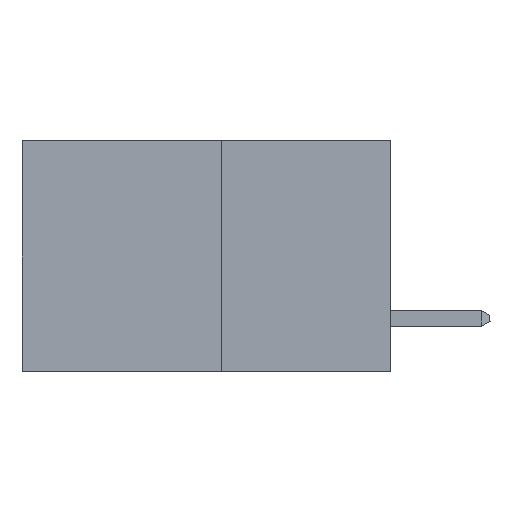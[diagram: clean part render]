
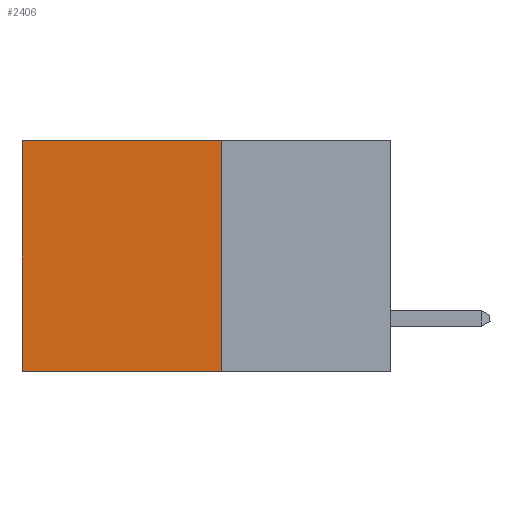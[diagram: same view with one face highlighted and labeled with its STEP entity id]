
A CAD part, left-side view. The second image highlights one B-rep face of the part: STEP entity #2406.
In plain terms, the highlighted planar face has unit normal (-1, 0, 0).
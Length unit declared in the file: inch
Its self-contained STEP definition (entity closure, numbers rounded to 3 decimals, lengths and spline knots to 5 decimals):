
#438 = VECTOR ( 'NONE', #16732, 39.37008 ) ;
#534 = VERTEX_POINT ( 'NONE', #14282 ) ;
#1206 = AXIS2_PLACEMENT_3D ( 'NONE', #14057, #15359, #7494 ) ;
#1408 = VECTOR ( 'NONE', #11348, 39.37008 ) ;
#2335 = CARTESIAN_POINT ( 'NONE',  ( 0.277, 0.27, -0.37 ) ) ;
#2406 = ADVANCED_FACE ( 'NONE', ( #8307 ), #11424, .F. ) ;
#2474 = ORIENTED_EDGE ( 'NONE', *, *, #8047, .T. ) ;
#2562 = DIRECTION ( 'NONE',  ( 0., 0., -1. ) ) ;
#2652 = VECTOR ( 'NONE', #2562, 39.37008 ) ;
#3081 = LINE ( 'NONE', #4979, #9716 ) ;
#3477 = VERTEX_POINT ( 'NONE', #4419 ) ;
#3604 = CARTESIAN_POINT ( 'NONE',  ( 0.277, 0.27, -0.37 ) ) ;
#3862 = CARTESIAN_POINT ( 'NONE',  ( 0.277, 0.59, -0.37 ) ) ;
#4419 = CARTESIAN_POINT ( 'NONE',  ( 0.277, 0.59, 0. ) ) ;
#4979 = CARTESIAN_POINT ( 'NONE',  ( 0.277, 0.59, -0.37 ) ) ;
#6320 = DIRECTION ( 'NONE',  ( 0., 0., -1. ) ) ;
#7274 = EDGE_CURVE ( 'NONE', #534, #3477, #8910, .T. ) ;
#7480 = VERTEX_POINT ( 'NONE', #3862 ) ;
#7494 = DIRECTION ( 'NONE',  ( 0., 0., -1. ) ) ;
#7549 = LINE ( 'NONE', #3604, #438 ) ;
#8047 = EDGE_CURVE ( 'NONE', #3477, #7480, #3081, .T. ) ;
#8205 = ORIENTED_EDGE ( 'NONE', *, *, #12122, .F. ) ;
#8307 = FACE_OUTER_BOUND ( 'NONE', #9210, .T. ) ;
#8910 = LINE ( 'NONE', #12678, #1408 ) ;
#9210 = EDGE_LOOP ( 'NONE', ( #2474, #15555, #8205, #13877 ) ) ;
#9716 = VECTOR ( 'NONE', #6320, 39.37008 ) ;
#11348 = DIRECTION ( 'NONE',  ( 0., 1., 0. ) ) ;
#11424 = PLANE ( 'NONE',  #1206 ) ;
#12122 = EDGE_CURVE ( 'NONE', #534, #15584, #12771, .T. ) ;
#12678 = CARTESIAN_POINT ( 'NONE',  ( 0.277, 0.27, 0. ) ) ;
#12771 = LINE ( 'NONE', #13070, #2652 ) ;
#13070 = CARTESIAN_POINT ( 'NONE',  ( 0.277, 0.27, -0.37 ) ) ;
#13482 = EDGE_CURVE ( 'NONE', #15584, #7480, #7549, .T. ) ;
#13877 = ORIENTED_EDGE ( 'NONE', *, *, #7274, .T. ) ;
#14057 = CARTESIAN_POINT ( 'NONE',  ( 0.277, 0.27, -0.37 ) ) ;
#14282 = CARTESIAN_POINT ( 'NONE',  ( 0.277, 0.27, 0. ) ) ;
#15359 = DIRECTION ( 'NONE',  ( 1., 0., 0. ) ) ;
#15555 = ORIENTED_EDGE ( 'NONE', *, *, #13482, .F. ) ;
#15584 = VERTEX_POINT ( 'NONE', #2335 ) ;
#16732 = DIRECTION ( 'NONE',  ( 0., 1., 0. ) ) ;
